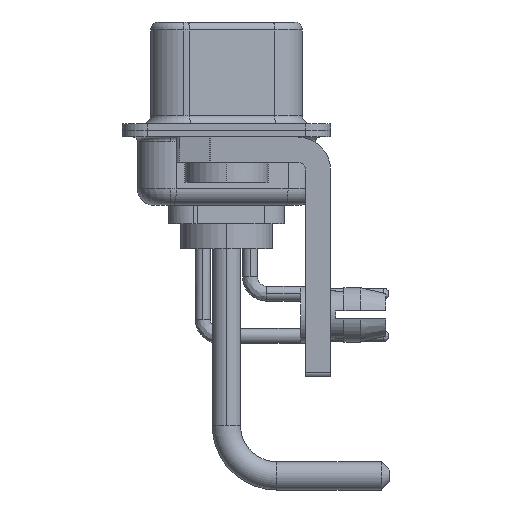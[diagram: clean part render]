
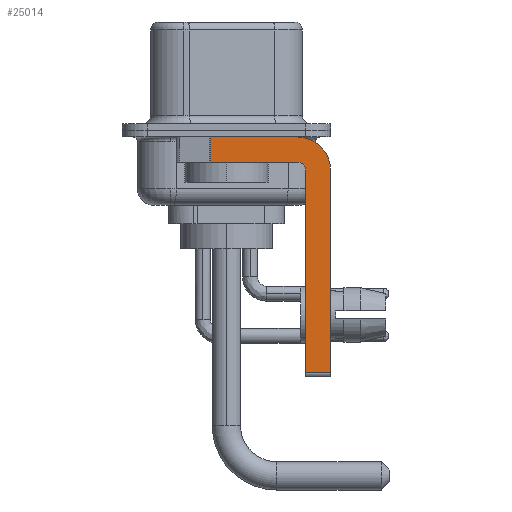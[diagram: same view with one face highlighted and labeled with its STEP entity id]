
A CAD part, left-side view. The second image highlights one B-rep face of the part: STEP entity #25014.
In plain terms, the highlighted planar face has unit normal (-1, 0, 0).
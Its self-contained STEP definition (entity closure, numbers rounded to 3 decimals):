
#150 = CARTESIAN_POINT ( 'NONE',  ( -2.9, 0.978, -1.9 ) ) ;
#1477 = VERTEX_POINT ( 'NONE', #15385 ) ;
#1702 = CIRCLE ( 'NONE', #6461, 2. ) ;
#1961 = DIRECTION ( 'NONE',  ( 0., -1., 0. ) ) ;
#2611 = VERTEX_POINT ( 'NONE', #21509 ) ;
#2706 = EDGE_CURVE ( 'NONE', #14707, #6439, #1702, .T. ) ;
#3114 = VERTEX_POINT ( 'NONE', #4514 ) ;
#3558 = CARTESIAN_POINT ( 'NONE',  ( -2.9, -4.75, -14.55 ) ) ;
#3745 = VERTEX_POINT ( 'NONE', #3558 ) ;
#4434 = DIRECTION ( 'NONE',  ( 1., 0., 0. ) ) ;
#4514 = CARTESIAN_POINT ( 'NONE',  ( -2.9, -6.25, -14.55 ) ) ;
#4982 = VECTOR ( 'NONE', #1961, 1000. ) ;
#5109 = AXIS2_PLACEMENT_3D ( 'NONE', #18823, #7401, #5182 ) ;
#5182 = DIRECTION ( 'NONE',  ( 0., 0., -1. ) ) ;
#6034 = LINE ( 'NONE', #26197, #28903 ) ;
#6184 = ORIENTED_EDGE ( 'NONE', *, *, #13000, .F. ) ;
#6308 = EDGE_LOOP ( 'NONE', ( #14908, #18957, #6184, #20569, #12164, #28879, #28477, #24818 ) ) ;
#6361 = CARTESIAN_POINT ( 'NONE',  ( -2.9, -4.25, -0.4 ) ) ;
#6382 = CARTESIAN_POINT ( 'NONE',  ( -2.9, -4.25, -2.4 ) ) ;
#6439 = VERTEX_POINT ( 'NONE', #16872 ) ;
#6461 = AXIS2_PLACEMENT_3D ( 'NONE', #6382, #4434, #11264 ) ;
#7401 = DIRECTION ( 'NONE',  ( 1., 0., 0. ) ) ;
#7702 = FACE_OUTER_BOUND ( 'NONE', #6308, .T. ) ;
#8197 = LINE ( 'NONE', #10720, #26269 ) ;
#9335 = VERTEX_POINT ( 'NONE', #24534 ) ;
#9700 = DIRECTION ( 'NONE',  ( 0., 0., 1. ) ) ;
#9856 = LINE ( 'NONE', #19178, #28355 ) ;
#10720 = CARTESIAN_POINT ( 'NONE',  ( -2.9, -4.25, -14.55 ) ) ;
#11204 = VECTOR ( 'NONE', #12049, 1000. ) ;
#11264 = DIRECTION ( 'NONE',  ( 0., 0., -1. ) ) ;
#12049 = DIRECTION ( 'NONE',  ( 0., 0., -1. ) ) ;
#12164 = ORIENTED_EDGE ( 'NONE', *, *, #26940, .F. ) ;
#12870 = DIRECTION ( 'NONE',  ( 0., 0., 1. ) ) ;
#13000 = EDGE_CURVE ( 'NONE', #2611, #9335, #16661, .T. ) ;
#14620 = CIRCLE ( 'NONE', #25022, 0.5 ) ;
#14707 = VERTEX_POINT ( 'NONE', #6361 ) ;
#14908 = ORIENTED_EDGE ( 'NONE', *, *, #20587, .F. ) ;
#15385 = CARTESIAN_POINT ( 'NONE',  ( -2.9, 0.978, -0.4 ) ) ;
#15438 = EDGE_CURVE ( 'NONE', #3745, #3114, #8197, .T. ) ;
#16661 = LINE ( 'NONE', #25701, #27971 ) ;
#16872 = CARTESIAN_POINT ( 'NONE',  ( -2.9, -6.25, -2.4 ) ) ;
#16964 = DIRECTION ( 'NONE',  ( 0., 1., 0. ) ) ;
#16972 = EDGE_CURVE ( 'NONE', #1477, #9335, #23019, .T. ) ;
#18823 = CARTESIAN_POINT ( 'NONE',  ( -2.9, -4.25, -2.4 ) ) ;
#18957 = ORIENTED_EDGE ( 'NONE', *, *, #16972, .T. ) ;
#19003 = EDGE_CURVE ( 'NONE', #20767, #2611, #14620, .T. ) ;
#19093 = EDGE_CURVE ( 'NONE', #6439, #3114, #9856, .T. ) ;
#19178 = CARTESIAN_POINT ( 'NONE',  ( -2.9, -6.25, -2.4 ) ) ;
#19789 = LINE ( 'NONE', #24951, #4982 ) ;
#20569 = ORIENTED_EDGE ( 'NONE', *, *, #19003, .F. ) ;
#20587 = EDGE_CURVE ( 'NONE', #1477, #14707, #19789, .T. ) ;
#20767 = VERTEX_POINT ( 'NONE', #27601 ) ;
#21509 = CARTESIAN_POINT ( 'NONE',  ( -2.9, -4.25, -1.9 ) ) ;
#21541 = DIRECTION ( 'NONE',  ( 0., 0., -1. ) ) ;
#22889 = CARTESIAN_POINT ( 'NONE',  ( -2.9, -4.25, -2.4 ) ) ;
#23019 = LINE ( 'NONE', #150, #11204 ) ;
#24534 = CARTESIAN_POINT ( 'NONE',  ( -2.9, 0.978, -1.9 ) ) ;
#24818 = ORIENTED_EDGE ( 'NONE', *, *, #2706, .F. ) ;
#24951 = CARTESIAN_POINT ( 'NONE',  ( -2.9, 3., -0.4 ) ) ;
#24975 = DIRECTION ( 'NONE',  ( -1., 0., 0. ) ) ;
#25014 = ADVANCED_FACE ( 'NONE', ( #7702 ), #28154, .F. ) ;
#25022 = AXIS2_PLACEMENT_3D ( 'NONE', #22889, #24975, #9700 ) ;
#25701 = CARTESIAN_POINT ( 'NONE',  ( -2.9, -4.25, -1.9 ) ) ;
#26135 = DIRECTION ( 'NONE',  ( 0., -1., 0. ) ) ;
#26197 = CARTESIAN_POINT ( 'NONE',  ( -2.9, -4.75, -14.8 ) ) ;
#26269 = VECTOR ( 'NONE', #26135, 1000. ) ;
#26940 = EDGE_CURVE ( 'NONE', #3745, #20767, #6034, .T. ) ;
#27601 = CARTESIAN_POINT ( 'NONE',  ( -2.9, -4.75, -2.4 ) ) ;
#27971 = VECTOR ( 'NONE', #16964, 1000. ) ;
#28154 = PLANE ( 'NONE',  #5109 ) ;
#28355 = VECTOR ( 'NONE', #21541, 1000. ) ;
#28477 = ORIENTED_EDGE ( 'NONE', *, *, #19093, .F. ) ;
#28879 = ORIENTED_EDGE ( 'NONE', *, *, #15438, .T. ) ;
#28903 = VECTOR ( 'NONE', #12870, 1000. ) ;
